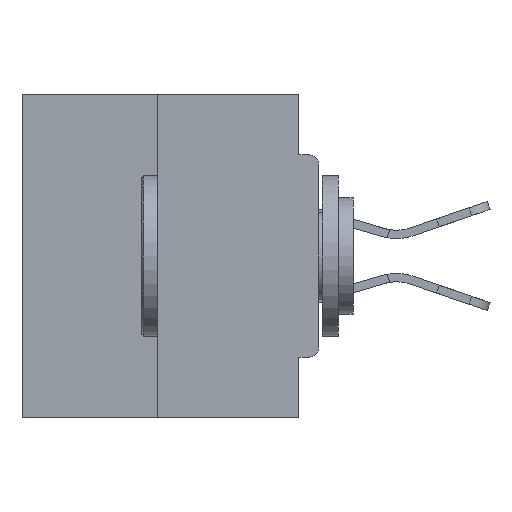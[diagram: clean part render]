
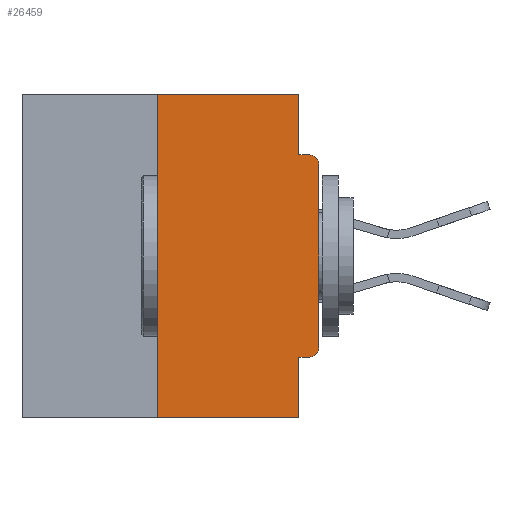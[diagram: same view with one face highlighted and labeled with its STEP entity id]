
A CAD part, left-side view. The second image highlights one B-rep face of the part: STEP entity #26459.
In plain terms, the highlighted planar face has unit normal (-1, 0, 0).
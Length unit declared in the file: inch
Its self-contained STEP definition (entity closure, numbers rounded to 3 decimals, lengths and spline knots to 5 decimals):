
#367 = VERTEX_POINT ( 'NONE', #33934 ) ;
#400 = EDGE_CURVE ( 'NONE', #37065, #3745, #23706, .T. ) ;
#575 = ORIENTED_EDGE ( 'NONE', *, *, #32330, .T. ) ;
#778 = LINE ( 'NONE', #26277, #13747 ) ;
#937 = CARTESIAN_POINT ( 'NONE',  ( 0., 0.46, 0. ) ) ;
#1004 = DIRECTION ( 'NONE',  ( 0., 1., 0. ) ) ;
#1175 = VECTOR ( 'NONE', #1004, 39.37008 ) ;
#1952 = VECTOR ( 'NONE', #5424, 39.37008 ) ;
#2640 = DIRECTION ( 'NONE',  ( -1., 0., 0. ) ) ;
#2906 = DIRECTION ( 'NONE',  ( 0., -1., 0. ) ) ;
#3745 = VERTEX_POINT ( 'NONE', #11587 ) ;
#4158 = CARTESIAN_POINT ( 'NONE',  ( 0., 0.46, 0. ) ) ;
#4263 = EDGE_CURVE ( 'NONE', #367, #36660, #778, .T. ) ;
#4698 = LINE ( 'NONE', #35869, #1952 ) ;
#5114 = CIRCLE ( 'NONE', #9069, 0.015 ) ;
#5155 = LINE ( 'NONE', #36118, #20060 ) ;
#5424 = DIRECTION ( 'NONE',  ( 0., 0., 1. ) ) ;
#6247 = ORIENTED_EDGE ( 'NONE', *, *, #4263, .T. ) ;
#6495 = DIRECTION ( 'NONE',  ( 0., 0., -1. ) ) ;
#6980 = PLANE ( 'NONE',  #15645 ) ;
#7202 = VERTEX_POINT ( 'NONE', #10604 ) ;
#8377 = DIRECTION ( 'NONE',  ( 0., -1., 0. ) ) ;
#8967 = VECTOR ( 'NONE', #16252, 39.37008 ) ;
#9051 = LINE ( 'NONE', #21524, #1175 ) ;
#9069 = AXIS2_PLACEMENT_3D ( 'NONE', #36968, #27789, #27911 ) ;
#9092 = ORIENTED_EDGE ( 'NONE', *, *, #27679, .F. ) ;
#9234 = DIRECTION ( 'NONE',  ( 0., 0., -1. ) ) ;
#9708 = ORIENTED_EDGE ( 'NONE', *, *, #38524, .F. ) ;
#10604 = CARTESIAN_POINT ( 'NONE',  ( 0., 0.031, -0.4065 ) ) ;
#10935 = VERTEX_POINT ( 'NONE', #35513 ) ;
#11587 = CARTESIAN_POINT ( 'NONE',  ( 0., 0., -0.3915 ) ) ;
#11946 = EDGE_CURVE ( 'NONE', #10935, #17503, #29922, .T. ) ;
#13508 = VERTEX_POINT ( 'NONE', #17792 ) ;
#13747 = VECTOR ( 'NONE', #2906, 39.37008 ) ;
#15645 = AXIS2_PLACEMENT_3D ( 'NONE', #937, #15860, #18585 ) ;
#15860 = DIRECTION ( 'NONE',  ( 1., 0., 0. ) ) ;
#16073 = EDGE_CURVE ( 'NONE', #13508, #10935, #25642, .T. ) ;
#16252 = DIRECTION ( 'NONE',  ( 0., -1., 0. ) ) ;
#17503 = VERTEX_POINT ( 'NONE', #28901 ) ;
#17792 = CARTESIAN_POINT ( 'NONE',  ( 0., 0.031, 0. ) ) ;
#18585 = DIRECTION ( 'NONE',  ( 0., 0., -1. ) ) ;
#18660 = ORIENTED_EDGE ( 'NONE', *, *, #35635, .T. ) ;
#18978 = ORIENTED_EDGE ( 'NONE', *, *, #22330, .F. ) ;
#19944 = AXIS2_PLACEMENT_3D ( 'NONE', #38227, #2640, #26390 ) ;
#20060 = VECTOR ( 'NONE', #6495, 39.37008 ) ;
#20233 = LINE ( 'NONE', #33010, #32304 ) ;
#21524 = CARTESIAN_POINT ( 'NONE',  ( 0., 0., -0.4065 ) ) ;
#22253 = ORIENTED_EDGE ( 'NONE', *, *, #16073, .F. ) ;
#22330 = EDGE_CURVE ( 'NONE', #24464, #13508, #32201, .T. ) ;
#22923 = CARTESIAN_POINT ( 'NONE',  ( 0., 0.031, -0.5 ) ) ;
#23706 = CIRCLE ( 'NONE', #19944, 0.015 ) ;
#24464 = VERTEX_POINT ( 'NONE', #27787 ) ;
#25340 = CARTESIAN_POINT ( 'NONE',  ( 0., 0., -0.0935 ) ) ;
#25642 = LINE ( 'NONE', #38079, #30786 ) ;
#26039 = VERTEX_POINT ( 'NONE', #27773 ) ;
#26277 = CARTESIAN_POINT ( 'NONE',  ( 0., 0.46, -0.5 ) ) ;
#26390 = DIRECTION ( 'NONE',  ( 0., 0., -1. ) ) ;
#26459 = ADVANCED_FACE ( 'NONE', ( #33276 ), #6980, .F. ) ;
#26508 = CARTESIAN_POINT ( 'NONE',  ( 0., 0.015, -0.4065 ) ) ;
#27679 = EDGE_CURVE ( 'NONE', #37065, #7202, #9051, .T. ) ;
#27773 = CARTESIAN_POINT ( 'NONE',  ( 0., 0., -0.1085 ) ) ;
#27787 = CARTESIAN_POINT ( 'NONE',  ( 0., 0.25, 0. ) ) ;
#27789 = DIRECTION ( 'NONE',  ( -1., 0., 0. ) ) ;
#27911 = DIRECTION ( 'NONE',  ( 0., 0., -1. ) ) ;
#28901 = CARTESIAN_POINT ( 'NONE',  ( 0., 0.015, -0.0935 ) ) ;
#29615 = ORIENTED_EDGE ( 'NONE', *, *, #31643, .F. ) ;
#29922 = LINE ( 'NONE', #25340, #8967 ) ;
#30786 = VECTOR ( 'NONE', #9234, 39.37008 ) ;
#31643 = EDGE_CURVE ( 'NONE', #367, #24464, #4698, .T. ) ;
#32201 = LINE ( 'NONE', #4158, #34500 ) ;
#32304 = VECTOR ( 'NONE', #38374, 39.37008 ) ;
#32330 = EDGE_CURVE ( 'NONE', #26039, #17503, #5114, .T. ) ;
#33010 = CARTESIAN_POINT ( 'NONE',  ( 0., 0., 0. ) ) ;
#33276 = FACE_OUTER_BOUND ( 'NONE', #35431, .T. ) ;
#33822 = ORIENTED_EDGE ( 'NONE', *, *, #400, .T. ) ;
#33934 = CARTESIAN_POINT ( 'NONE',  ( 0., 0.25, -0.5 ) ) ;
#33975 = ORIENTED_EDGE ( 'NONE', *, *, #11946, .F. ) ;
#34500 = VECTOR ( 'NONE', #8377, 39.37008 ) ;
#35431 = EDGE_LOOP ( 'NONE', ( #18978, #29615, #6247, #9708, #9092, #33822, #18660, #575, #33975, #22253 ) ) ;
#35513 = CARTESIAN_POINT ( 'NONE',  ( 0., 0.031, -0.0935 ) ) ;
#35635 = EDGE_CURVE ( 'NONE', #3745, #26039, #20233, .T. ) ;
#35869 = CARTESIAN_POINT ( 'NONE',  ( 0., 0.25, 0. ) ) ;
#36118 = CARTESIAN_POINT ( 'NONE',  ( 0., 0.031, -0.5 ) ) ;
#36660 = VERTEX_POINT ( 'NONE', #22923 ) ;
#36968 = CARTESIAN_POINT ( 'NONE',  ( 0., 0.015, -0.1085 ) ) ;
#37065 = VERTEX_POINT ( 'NONE', #26508 ) ;
#38079 = CARTESIAN_POINT ( 'NONE',  ( 0., 0.031, 0. ) ) ;
#38227 = CARTESIAN_POINT ( 'NONE',  ( 0., 0.015, -0.3915 ) ) ;
#38374 = DIRECTION ( 'NONE',  ( 0., 0., 1. ) ) ;
#38524 = EDGE_CURVE ( 'NONE', #7202, #36660, #5155, .T. ) ;
